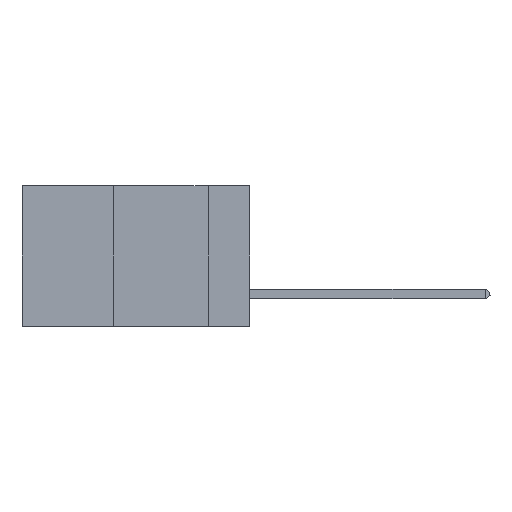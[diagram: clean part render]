
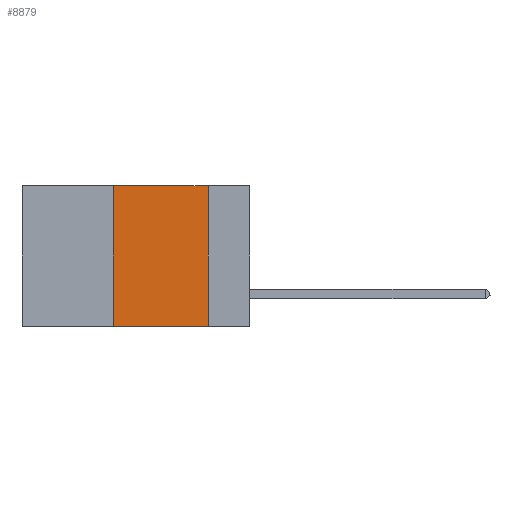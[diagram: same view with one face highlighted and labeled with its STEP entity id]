
A CAD part, left-side view. The second image highlights one B-rep face of the part: STEP entity #8879.
In plain terms, the highlighted planar face has unit normal (-1, 0, 0).
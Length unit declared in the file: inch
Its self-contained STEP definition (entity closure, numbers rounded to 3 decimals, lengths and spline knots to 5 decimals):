
#926 = CARTESIAN_POINT ( 'NONE',  ( 0., 0.6, 0. ) ) ;
#1020 = EDGE_CURVE ( 'NONE', #13171, #2464, #16429, .T. ) ;
#1141 = CARTESIAN_POINT ( 'NONE',  ( 0., 0.6, -0.37 ) ) ;
#1163 = DIRECTION ( 'NONE',  ( 1., 0., 0. ) ) ;
#2395 = LINE ( 'NONE', #8899, #7306 ) ;
#2464 = VERTEX_POINT ( 'NONE', #13763 ) ;
#2841 = DIRECTION ( 'NONE',  ( 0., 0., 1. ) ) ;
#3316 = PLANE ( 'NONE',  #17490 ) ;
#3887 = FACE_OUTER_BOUND ( 'NONE', #9292, .T. ) ;
#3918 = DIRECTION ( 'NONE',  ( 0., 0., -1. ) ) ;
#5314 = EDGE_CURVE ( 'NONE', #13171, #13512, #14559, .T. ) ;
#6508 = CARTESIAN_POINT ( 'NONE',  ( 0., 0.11, 0. ) ) ;
#7026 = LINE ( 'NONE', #6508, #11031 ) ;
#7306 = VECTOR ( 'NONE', #14037, 39.37008 ) ;
#8427 = EDGE_CURVE ( 'NONE', #13512, #9668, #2395, .T. ) ;
#8701 = ORIENTED_EDGE ( 'NONE', *, *, #5314, .F. ) ;
#8879 = ADVANCED_FACE ( 'NONE', ( #3887 ), #3316, .F. ) ;
#8899 = CARTESIAN_POINT ( 'NONE',  ( 0., 0.6, 0. ) ) ;
#9163 = DIRECTION ( 'NONE',  ( 0., 0., -1. ) ) ;
#9292 = EDGE_LOOP ( 'NONE', ( #14572, #14453, #8701, #15457 ) ) ;
#9668 = VERTEX_POINT ( 'NONE', #15106 ) ;
#10964 = VECTOR ( 'NONE', #2841, 39.37008 ) ;
#11031 = VECTOR ( 'NONE', #9163, 39.37008 ) ;
#11109 = CARTESIAN_POINT ( 'NONE',  ( 0., 0.36, -0.37 ) ) ;
#11380 = VECTOR ( 'NONE', #17257, 39.37008 ) ;
#12254 = CARTESIAN_POINT ( 'NONE',  ( 0., 0.36, 0. ) ) ;
#12570 = EDGE_CURVE ( 'NONE', #9668, #2464, #7026, .T. ) ;
#13171 = VERTEX_POINT ( 'NONE', #11109 ) ;
#13512 = VERTEX_POINT ( 'NONE', #14262 ) ;
#13763 = CARTESIAN_POINT ( 'NONE',  ( 0., 0.11, -0.37 ) ) ;
#14037 = DIRECTION ( 'NONE',  ( 0., -1., 0. ) ) ;
#14262 = CARTESIAN_POINT ( 'NONE',  ( 0., 0.36, 0. ) ) ;
#14453 = ORIENTED_EDGE ( 'NONE', *, *, #8427, .F. ) ;
#14559 = LINE ( 'NONE', #12254, #10964 ) ;
#14572 = ORIENTED_EDGE ( 'NONE', *, *, #12570, .F. ) ;
#15106 = CARTESIAN_POINT ( 'NONE',  ( 0., 0.11, 0. ) ) ;
#15457 = ORIENTED_EDGE ( 'NONE', *, *, #1020, .T. ) ;
#16429 = LINE ( 'NONE', #1141, #11380 ) ;
#17257 = DIRECTION ( 'NONE',  ( 0., -1., 0. ) ) ;
#17490 = AXIS2_PLACEMENT_3D ( 'NONE', #926, #1163, #3918 ) ;
